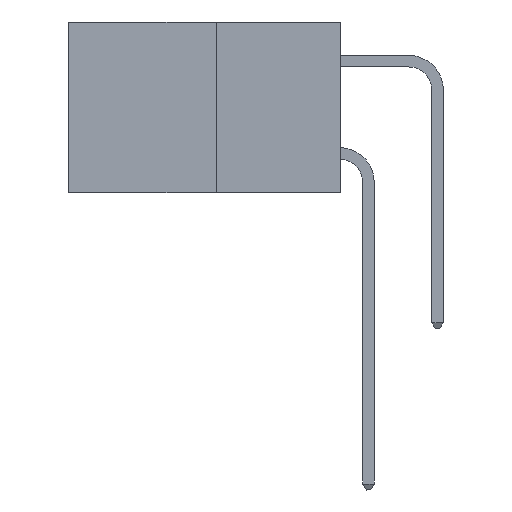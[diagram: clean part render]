
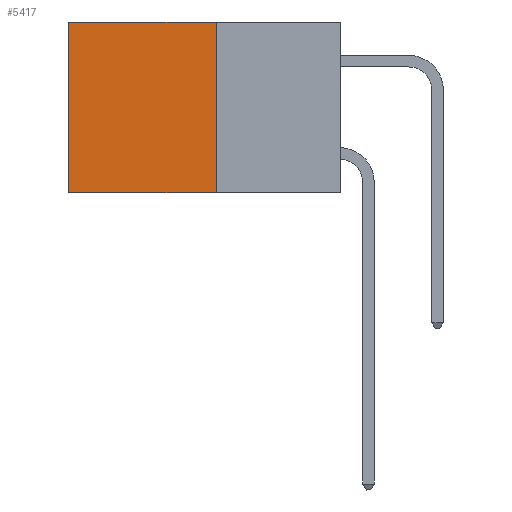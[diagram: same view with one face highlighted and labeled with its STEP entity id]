
A CAD part, left-side view. The second image highlights one B-rep face of the part: STEP entity #5417.
In plain terms, the highlighted planar face has unit normal (-1, 0, 0).
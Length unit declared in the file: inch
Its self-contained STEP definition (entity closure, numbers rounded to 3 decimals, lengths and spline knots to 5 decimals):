
#101 = ORIENTED_EDGE ( 'NONE', *, *, #1082, .T. ) ;
#463 = ORIENTED_EDGE ( 'NONE', *, *, #9706, .F. ) ;
#1002 = LINE ( 'NONE', #4577, #11279 ) ;
#1082 = EDGE_CURVE ( 'NONE', #6792, #2413, #1002, .T. ) ;
#1984 = CARTESIAN_POINT ( 'NONE',  ( 0.277, 0.27, -0.37 ) ) ;
#2413 = VERTEX_POINT ( 'NONE', #2708 ) ;
#2708 = CARTESIAN_POINT ( 'NONE',  ( 0.277, 0.59, -0.37 ) ) ;
#3042 = PLANE ( 'NONE',  #18948 ) ;
#3672 = LINE ( 'NONE', #26128, #19310 ) ;
#4063 = DIRECTION ( 'NONE',  ( 0., 1., 0. ) ) ;
#4577 = CARTESIAN_POINT ( 'NONE',  ( 0.277, 0.59, -0.37 ) ) ;
#5270 = LINE ( 'NONE', #9225, #10714 ) ;
#5417 = ADVANCED_FACE ( 'NONE', ( #9037 ), #3042, .F. ) ;
#6792 = VERTEX_POINT ( 'NONE', #9568 ) ;
#7187 = DIRECTION ( 'NONE',  ( 1., 0., 0. ) ) ;
#8819 = ORIENTED_EDGE ( 'NONE', *, *, #10565, .F. ) ;
#9037 = FACE_OUTER_BOUND ( 'NONE', #13364, .T. ) ;
#9225 = CARTESIAN_POINT ( 'NONE',  ( 0.277, 0.27, -0.37 ) ) ;
#9568 = CARTESIAN_POINT ( 'NONE',  ( 0.277, 0.59, 0. ) ) ;
#9706 = EDGE_CURVE ( 'NONE', #18480, #9741, #5270, .T. ) ;
#9741 = VERTEX_POINT ( 'NONE', #15342 ) ;
#10565 = EDGE_CURVE ( 'NONE', #9741, #2413, #17344, .T. ) ;
#10714 = VECTOR ( 'NONE', #23391, 39.37008 ) ;
#11279 = VECTOR ( 'NONE', #23099, 39.37008 ) ;
#13193 = ORIENTED_EDGE ( 'NONE', *, *, #14894, .T. ) ;
#13364 = EDGE_LOOP ( 'NONE', ( #101, #8819, #463, #13193 ) ) ;
#14073 = DIRECTION ( 'NONE',  ( 0., 1., 0. ) ) ;
#14894 = EDGE_CURVE ( 'NONE', #18480, #6792, #3672, .T. ) ;
#15342 = CARTESIAN_POINT ( 'NONE',  ( 0.277, 0.27, -0.37 ) ) ;
#17344 = LINE ( 'NONE', #1984, #22080 ) ;
#18480 = VERTEX_POINT ( 'NONE', #20488 ) ;
#18948 = AXIS2_PLACEMENT_3D ( 'NONE', #25308, #7187, #21444 ) ;
#19310 = VECTOR ( 'NONE', #14073, 39.37008 ) ;
#20488 = CARTESIAN_POINT ( 'NONE',  ( 0.277, 0.27, 0. ) ) ;
#21444 = DIRECTION ( 'NONE',  ( 0., 0., -1. ) ) ;
#22080 = VECTOR ( 'NONE', #4063, 39.37008 ) ;
#23099 = DIRECTION ( 'NONE',  ( 0., 0., -1. ) ) ;
#23391 = DIRECTION ( 'NONE',  ( 0., 0., -1. ) ) ;
#25308 = CARTESIAN_POINT ( 'NONE',  ( 0.277, 0.27, -0.37 ) ) ;
#26128 = CARTESIAN_POINT ( 'NONE',  ( 0.277, 0.27, 0. ) ) ;
